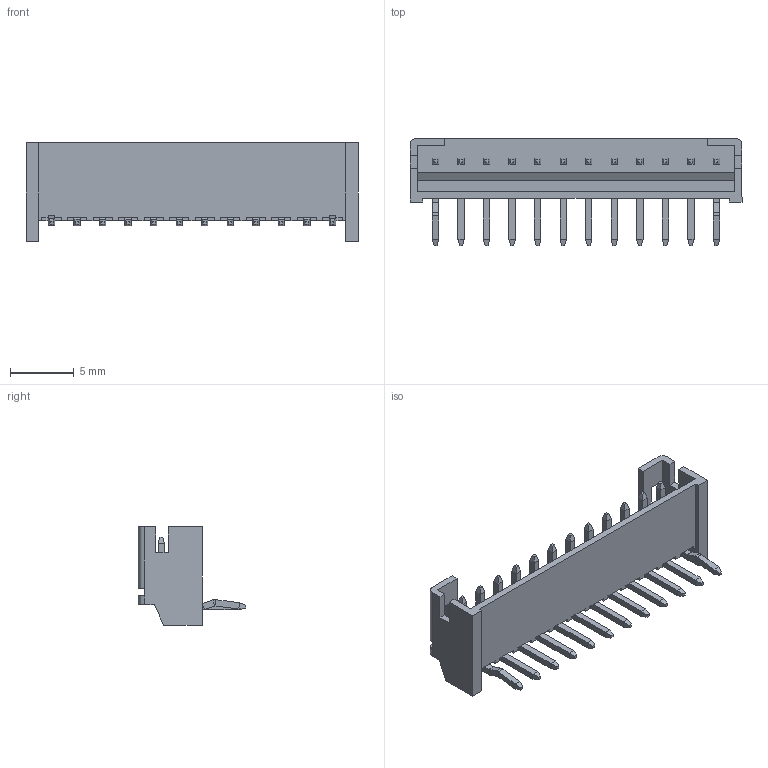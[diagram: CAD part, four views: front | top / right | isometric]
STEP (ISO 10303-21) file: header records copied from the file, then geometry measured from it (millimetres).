
FILE_DESCRIPTION (( 'STEP AP203' ), '1' );
FILE_NAME ('140-512-415-000.STEP', '2020-03-31T19:45:35', ( '' ), ( '' ), 'SwSTEP 2.0', 'SolidWorks 2016', '' );
FILE_SCHEMA (( 'CONFIG_CONTROL_DESIGN' ));
Length unit declared in the file: millimetre
Products named in the file (4): RA Contact_Str; RA Contact_Kink; 140-512-415-000; RA Housing_512
Assembly tree (13 placements, depth 2):
  140-512-415-000
    RA Housing_512
    RA Contact_Kink  x2
    RA Contact_Str  x10
Bounding box: 26 x 8.41 x 7.7 mm (x, y, z)
Volume: 299.1 mm3; surface area: 1103.9 mm2
Topology: 13 solids, 13 shells, 439 faces, 1017 edges, 602 vertices
Faces by surface type: plane 403, cylinder 36
Entity records: 6957 total; most frequent: CARTESIAN_POINT 1110, ORIENTED_EDGE 1090, DIRECTION 1007, EDGE_CURVE 545, LINE 521, VECTOR 521, VERTEX_POINT 346, AXIS2_PLACEMENT_3D 243
